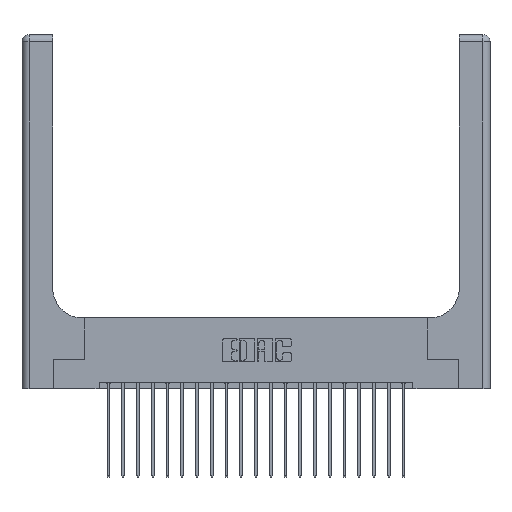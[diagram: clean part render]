
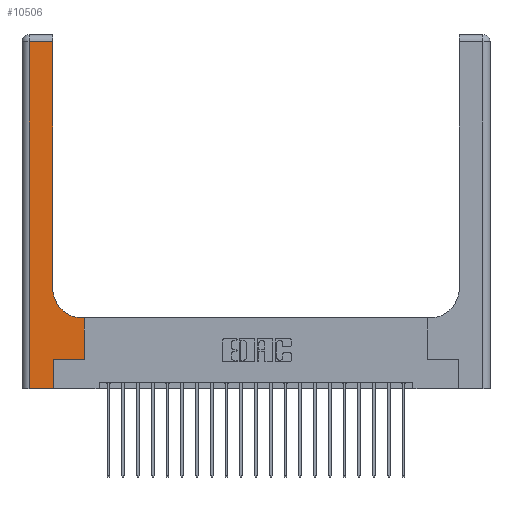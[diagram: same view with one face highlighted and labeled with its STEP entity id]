
A CAD part, top view. The second image highlights one B-rep face of the part: STEP entity #10506.
In plain terms, the highlighted planar face has unit normal (0, 0, 1).
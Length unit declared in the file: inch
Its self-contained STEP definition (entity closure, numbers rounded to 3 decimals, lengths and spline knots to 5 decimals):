
#265 = ORIENTED_EDGE ( 'NONE', *, *, #6912, .T. ) ;
#858 = VERTEX_POINT ( 'NONE', #13318 ) ;
#1070 = CARTESIAN_POINT ( 'NONE',  ( 0.528, 0.25, 0.37 ) ) ;
#1382 = LINE ( 'NONE', #8959, #13442 ) ;
#1781 = EDGE_CURVE ( 'NONE', #12874, #20735, #11255, .T. ) ;
#1903 = LINE ( 'NONE', #13567, #5835 ) ;
#1969 = DIRECTION ( 'NONE',  ( -1., 0., 0. ) ) ;
#2442 = LINE ( 'NONE', #5466, #11635 ) ;
#2444 = DIRECTION ( 'NONE',  ( 0., -1., 0. ) ) ;
#2855 = CARTESIAN_POINT ( 'NONE',  ( 0.265, 0., 0.37 ) ) ;
#3365 = LINE ( 'NONE', #14175, #11212 ) ;
#3538 = DIRECTION ( 'NONE',  ( 1., 0., 0. ) ) ;
#3634 = ORIENTED_EDGE ( 'NONE', *, *, #20787, .T. ) ;
#3635 = EDGE_CURVE ( 'NONE', #12932, #21680, #3365, .T. ) ;
#3779 = PLANE ( 'NONE',  #5717 ) ;
#4421 = LINE ( 'NONE', #8311, #20996 ) ;
#5218 = CARTESIAN_POINT ( 'NONE',  ( 0.51, 0.6, 0.37 ) ) ;
#5424 = CARTESIAN_POINT ( 'NONE',  ( 0.26, 2.94, 0.37 ) ) ;
#5464 = CARTESIAN_POINT ( 'NONE',  ( 0.26, 0.85, 0.37 ) ) ;
#5466 = CARTESIAN_POINT ( 'NONE',  ( 0., 2.94, 0.37 ) ) ;
#5717 = AXIS2_PLACEMENT_3D ( 'NONE', #12200, #7066, #8746 ) ;
#5835 = VECTOR ( 'NONE', #3538, 39.37008 ) ;
#6912 = EDGE_CURVE ( 'NONE', #20735, #7486, #17029, .T. ) ;
#7066 = DIRECTION ( 'NONE',  ( 0., 0., -1. ) ) ;
#7486 = VERTEX_POINT ( 'NONE', #5464 ) ;
#8311 = CARTESIAN_POINT ( 'NONE',  ( 0.528, 0.25, 0.37 ) ) ;
#8585 = CARTESIAN_POINT ( 'NONE',  ( 0.265, 0.25, 0.37 ) ) ;
#8662 = DIRECTION ( 'NONE',  ( 1., 0., 0. ) ) ;
#8746 = DIRECTION ( 'NONE',  ( -1., 0., 0. ) ) ;
#8809 = CARTESIAN_POINT ( 'NONE',  ( 0.06, 0., 0.37 ) ) ;
#8894 = VECTOR ( 'NONE', #16496, 39.37008 ) ;
#8959 = CARTESIAN_POINT ( 'NONE',  ( 0.26, 3., 0.37 ) ) ;
#9125 = ORIENTED_EDGE ( 'NONE', *, *, #19157, .T. ) ;
#9191 = CARTESIAN_POINT ( 'NONE',  ( 0.265, 0., 0.37 ) ) ;
#9558 = ORIENTED_EDGE ( 'NONE', *, *, #21642, .T. ) ;
#10099 = LINE ( 'NONE', #2855, #20616 ) ;
#10167 = VERTEX_POINT ( 'NONE', #1070 ) ;
#10506 = ADVANCED_FACE ( 'NONE', ( #12884 ), #3779, .F. ) ;
#10699 = DIRECTION ( 'NONE',  ( 0., 0., -1. ) ) ;
#11018 = ORIENTED_EDGE ( 'NONE', *, *, #3635, .T. ) ;
#11081 = ORIENTED_EDGE ( 'NONE', *, *, #19624, .T. ) ;
#11212 = VECTOR ( 'NONE', #2444, 39.37008 ) ;
#11255 = LINE ( 'NONE', #11405, #8894 ) ;
#11405 = CARTESIAN_POINT ( 'NONE',  ( 0.26, 0.6, 0.37 ) ) ;
#11635 = VECTOR ( 'NONE', #1969, 39.37008 ) ;
#12166 = CARTESIAN_POINT ( 'NONE',  ( 0.51, 0.85, 0.37 ) ) ;
#12200 = CARTESIAN_POINT ( 'NONE',  ( 0., 3., 0.37 ) ) ;
#12874 = VERTEX_POINT ( 'NONE', #21313 ) ;
#12884 = FACE_OUTER_BOUND ( 'NONE', #21165, .T. ) ;
#12932 = VERTEX_POINT ( 'NONE', #14911 ) ;
#13318 = CARTESIAN_POINT ( 'NONE',  ( 0.265, 0.25, 0.37 ) ) ;
#13442 = VECTOR ( 'NONE', #15806, 39.37008 ) ;
#13567 = CARTESIAN_POINT ( 'NONE',  ( 0., 0., 0.37 ) ) ;
#13852 = ORIENTED_EDGE ( 'NONE', *, *, #17533, .T. ) ;
#14137 = EDGE_CURVE ( 'NONE', #10167, #12874, #4421, .T. ) ;
#14175 = CARTESIAN_POINT ( 'NONE',  ( 0.06, 3., 0.37 ) ) ;
#14659 = DIRECTION ( 'NONE',  ( 0., 1., 0. ) ) ;
#14911 = CARTESIAN_POINT ( 'NONE',  ( 0.06, 2.94, 0.37 ) ) ;
#14953 = VERTEX_POINT ( 'NONE', #5424 ) ;
#15806 = DIRECTION ( 'NONE',  ( 0., 1., 0. ) ) ;
#16367 = LINE ( 'NONE', #8585, #17409 ) ;
#16496 = DIRECTION ( 'NONE',  ( -1., 0., 0. ) ) ;
#17029 = CIRCLE ( 'NONE', #20891, 0.25 ) ;
#17409 = VECTOR ( 'NONE', #8662, 39.37008 ) ;
#17533 = EDGE_CURVE ( 'NONE', #14953, #12932, #2442, .T. ) ;
#17880 = ORIENTED_EDGE ( 'NONE', *, *, #1781, .T. ) ;
#18763 = DIRECTION ( 'NONE',  ( 1., 0., 0. ) ) ;
#18830 = VERTEX_POINT ( 'NONE', #9191 ) ;
#19157 = EDGE_CURVE ( 'NONE', #858, #10167, #16367, .T. ) ;
#19624 = EDGE_CURVE ( 'NONE', #18830, #858, #10099, .T. ) ;
#20070 = DIRECTION ( 'NONE',  ( 0., 1., 0. ) ) ;
#20271 = ORIENTED_EDGE ( 'NONE', *, *, #14137, .T. ) ;
#20616 = VECTOR ( 'NONE', #14659, 39.37008 ) ;
#20735 = VERTEX_POINT ( 'NONE', #5218 ) ;
#20787 = EDGE_CURVE ( 'NONE', #21680, #18830, #1903, .T. ) ;
#20891 = AXIS2_PLACEMENT_3D ( 'NONE', #12166, #10699, #18763 ) ;
#20996 = VECTOR ( 'NONE', #20070, 39.37008 ) ;
#21165 = EDGE_LOOP ( 'NONE', ( #9558, #13852, #11018, #3634, #11081, #9125, #20271, #17880, #265 ) ) ;
#21313 = CARTESIAN_POINT ( 'NONE',  ( 0.528, 0.6, 0.37 ) ) ;
#21642 = EDGE_CURVE ( 'NONE', #7486, #14953, #1382, .T. ) ;
#21680 = VERTEX_POINT ( 'NONE', #8809 ) ;
